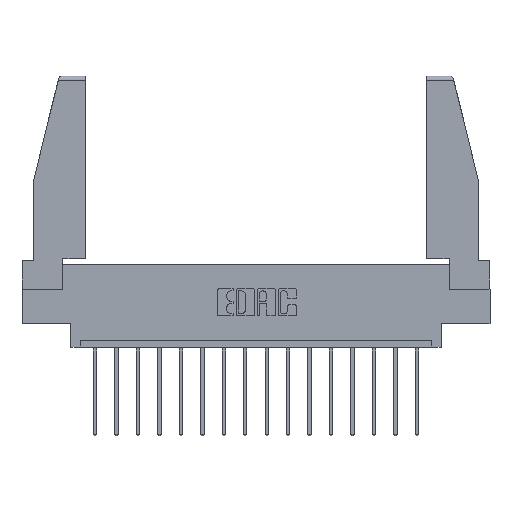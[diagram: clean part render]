
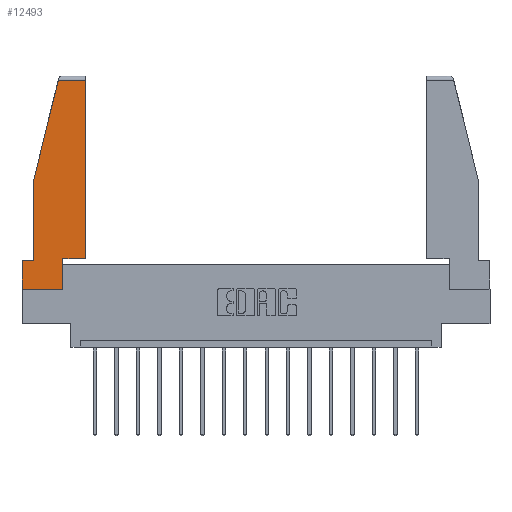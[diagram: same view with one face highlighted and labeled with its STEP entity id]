
A CAD part, top view. The second image highlights one B-rep face of the part: STEP entity #12493.
In plain terms, the highlighted planar face has unit normal (0, 0, 1).
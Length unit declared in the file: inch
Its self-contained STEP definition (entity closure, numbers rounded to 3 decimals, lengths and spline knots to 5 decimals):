
#446 = VECTOR ( 'NONE', #6666, 39.37008 ) ;
#514 = VECTOR ( 'NONE', #4769, 39.37008 ) ;
#572 = DIRECTION ( 'NONE',  ( -1., 0., 0. ) ) ;
#775 = DIRECTION ( 'NONE',  ( 0., 1., 0. ) ) ;
#967 = CARTESIAN_POINT ( 'NONE',  ( 0., 0., 0. ) ) ;
#1362 = ORIENTED_EDGE ( 'NONE', *, *, #7167, .T. ) ;
#1364 = LINE ( 'NONE', #11614, #3684 ) ;
#2315 = VERTEX_POINT ( 'NONE', #7373 ) ;
#2573 = LINE ( 'NONE', #10518, #2782 ) ;
#2656 = EDGE_CURVE ( 'NONE', #2726, #9971, #16458, .T. ) ;
#2726 = VERTEX_POINT ( 'NONE', #8810 ) ;
#2782 = VECTOR ( 'NONE', #4924, 39.37008 ) ;
#2998 = ORIENTED_EDGE ( 'NONE', *, *, #15992, .T. ) ;
#3238 = LINE ( 'NONE', #12852, #12953 ) ;
#3293 = ORIENTED_EDGE ( 'NONE', *, *, #5615, .T. ) ;
#3325 = FACE_OUTER_BOUND ( 'NONE', #14283, .T. ) ;
#3460 = LINE ( 'NONE', #13806, #4111 ) ;
#3684 = VECTOR ( 'NONE', #5994, 39.37008 ) ;
#3847 = VERTEX_POINT ( 'NONE', #7509 ) ;
#4111 = VECTOR ( 'NONE', #8092, 39.37008 ) ;
#4645 = DIRECTION ( 'NONE',  ( 0., -1., 0. ) ) ;
#4760 = CARTESIAN_POINT ( 'NONE',  ( 0., 0.21, 0. ) ) ;
#4769 = DIRECTION ( 'NONE',  ( 1., 0., 0. ) ) ;
#4799 = ORIENTED_EDGE ( 'NONE', *, *, #2656, .T. ) ;
#4924 = DIRECTION ( 'NONE',  ( 0., -1., 0. ) ) ;
#5615 = EDGE_CURVE ( 'NONE', #12755, #3847, #1364, .T. ) ;
#5643 = EDGE_CURVE ( 'NONE', #8467, #12755, #7844, .T. ) ;
#5994 = DIRECTION ( 'NONE',  ( 0., 1., 0. ) ) ;
#6468 = CARTESIAN_POINT ( 'NONE',  ( 0.297, 0., 0. ) ) ;
#6666 = DIRECTION ( 'NONE',  ( -0.239, -0.971, 0. ) ) ;
#6667 = ORIENTED_EDGE ( 'NONE', *, *, #17302, .T. ) ;
#6863 = EDGE_CURVE ( 'NONE', #10808, #2726, #3460, .T. ) ;
#7167 = EDGE_CURVE ( 'NONE', #3847, #8548, #3238, .T. ) ;
#7203 = DIRECTION ( 'NONE',  ( 0., 0., 1. ) ) ;
#7373 = CARTESIAN_POINT ( 'NONE',  ( 0.297, 0., 0. ) ) ;
#7470 = CARTESIAN_POINT ( 'NONE',  ( 0.297, 0.223, 0. ) ) ;
#7509 = CARTESIAN_POINT ( 'NONE',  ( 0.461, 1.52, 0. ) ) ;
#7730 = CARTESIAN_POINT ( 'NONE',  ( 0.086, 0.8, 0. ) ) ;
#7844 = LINE ( 'NONE', #7470, #514 ) ;
#8037 = ORIENTED_EDGE ( 'NONE', *, *, #5643, .T. ) ;
#8092 = DIRECTION ( 'NONE',  ( -1., 0., 0. ) ) ;
#8379 = VECTOR ( 'NONE', #10810, 39.37008 ) ;
#8415 = LINE ( 'NONE', #14915, #8379 ) ;
#8467 = VERTEX_POINT ( 'NONE', #13671 ) ;
#8548 = VERTEX_POINT ( 'NONE', #12743 ) ;
#8810 = CARTESIAN_POINT ( 'NONE',  ( 0., 0.21, 0. ) ) ;
#9971 = VERTEX_POINT ( 'NONE', #967 ) ;
#10518 = CARTESIAN_POINT ( 'NONE',  ( 0.086, 0.8, 0. ) ) ;
#10564 = CARTESIAN_POINT ( 'NONE',  ( 0.086, 0.21, 0. ) ) ;
#10582 = VERTEX_POINT ( 'NONE', #7730 ) ;
#10808 = VERTEX_POINT ( 'NONE', #10564 ) ;
#10810 = DIRECTION ( 'NONE',  ( 1., 0., 0. ) ) ;
#11614 = CARTESIAN_POINT ( 'NONE',  ( 0.461, 0.223, 0. ) ) ;
#11868 = AXIS2_PLACEMENT_3D ( 'NONE', #16946, #7203, #17008 ) ;
#12493 = ADVANCED_FACE ( 'NONE', ( #3325 ), #14519, .T. ) ;
#12743 = CARTESIAN_POINT ( 'NONE',  ( 0.2636, 1.52, 0. ) ) ;
#12755 = VERTEX_POINT ( 'NONE', #17465 ) ;
#12791 = LINE ( 'NONE', #6468, #16068 ) ;
#12852 = CARTESIAN_POINT ( 'NONE',  ( 0., 1.52, 0. ) ) ;
#12946 = VECTOR ( 'NONE', #4645, 39.37008 ) ;
#12953 = VECTOR ( 'NONE', #572, 39.37008 ) ;
#13671 = CARTESIAN_POINT ( 'NONE',  ( 0.297, 0.223, 0. ) ) ;
#13803 = CARTESIAN_POINT ( 'NONE',  ( 0.271, 1.55, 0. ) ) ;
#13806 = CARTESIAN_POINT ( 'NONE',  ( 0., 0.21, 0. ) ) ;
#14105 = EDGE_CURVE ( 'NONE', #2315, #8467, #12791, .T. ) ;
#14283 = EDGE_LOOP ( 'NONE', ( #3293, #1362, #6667, #2998, #14912, #4799, #17745, #15447, #8037 ) ) ;
#14519 = PLANE ( 'NONE',  #11868 ) ;
#14912 = ORIENTED_EDGE ( 'NONE', *, *, #6863, .T. ) ;
#14915 = CARTESIAN_POINT ( 'NONE',  ( 0., 0., 0. ) ) ;
#15447 = ORIENTED_EDGE ( 'NONE', *, *, #14105, .T. ) ;
#15990 = LINE ( 'NONE', #13803, #446 ) ;
#15992 = EDGE_CURVE ( 'NONE', #10582, #10808, #2573, .T. ) ;
#16068 = VECTOR ( 'NONE', #775, 39.37008 ) ;
#16171 = EDGE_CURVE ( 'NONE', #9971, #2315, #8415, .T. ) ;
#16458 = LINE ( 'NONE', #4760, #12946 ) ;
#16946 = CARTESIAN_POINT ( 'NONE',  ( 0., 0., 0. ) ) ;
#17008 = DIRECTION ( 'NONE',  ( 1., 0., 0. ) ) ;
#17302 = EDGE_CURVE ( 'NONE', #8548, #10582, #15990, .T. ) ;
#17465 = CARTESIAN_POINT ( 'NONE',  ( 0.461, 0.223, 0. ) ) ;
#17745 = ORIENTED_EDGE ( 'NONE', *, *, #16171, .T. ) ;
